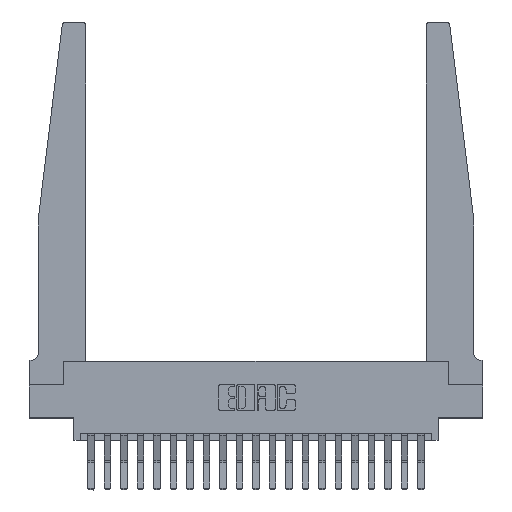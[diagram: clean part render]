
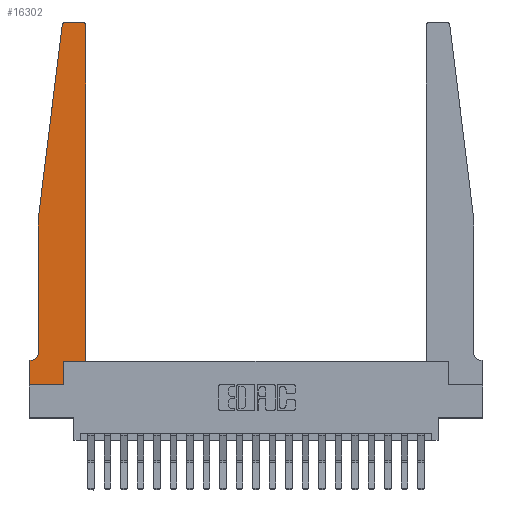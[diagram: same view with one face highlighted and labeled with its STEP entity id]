
A CAD part, top view. The second image highlights one B-rep face of the part: STEP entity #16302.
In plain terms, the highlighted planar face has unit normal (0, 0, 1).
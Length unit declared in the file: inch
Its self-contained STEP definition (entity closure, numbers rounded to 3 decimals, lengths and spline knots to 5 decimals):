
#2 = CARTESIAN_POINT ( 'NONE',  ( 0.395, 2.72, 0.37 ) ) ;
#70 = ORIENTED_EDGE ( 'NONE', *, *, #5399, .T. ) ;
#332 = CARTESIAN_POINT ( 'NONE',  ( 0.015, 0.2375, 0.37 ) ) ;
#385 = DIRECTION ( 'NONE',  ( 1., 0., 0. ) ) ;
#706 = VECTOR ( 'NONE', #16317, 39.37008 ) ;
#836 = CARTESIAN_POINT ( 'NONE',  ( 0.065, 0.2375, 0.37 ) ) ;
#853 = DIRECTION ( 'NONE',  ( 0., -1., 0. ) ) ;
#1120 = LINE ( 'NONE', #12809, #9482 ) ;
#1611 = VERTEX_POINT ( 'NONE', #3954 ) ;
#1660 = DIRECTION ( 'NONE',  ( 1., 0., 0. ) ) ;
#1911 = VERTEX_POINT ( 'NONE', #16457 ) ;
#1987 = DIRECTION ( 'NONE',  ( -1., 0., 0. ) ) ;
#2037 = AXIS2_PLACEMENT_3D ( 'NONE', #4890, #6555, #18270 ) ;
#2272 = ORIENTED_EDGE ( 'NONE', *, *, #21224, .T. ) ;
#2497 = ORIENTED_EDGE ( 'NONE', *, *, #7414, .T. ) ;
#2918 = CARTESIAN_POINT ( 'NONE',  ( 0.25, 2.75, 0.37 ) ) ;
#2957 = AXIS2_PLACEMENT_3D ( 'NONE', #2, #11694, #1660 ) ;
#3828 = CARTESIAN_POINT ( 'NONE',  ( 0., 0., 0.37 ) ) ;
#3954 = CARTESIAN_POINT ( 'NONE',  ( 0.425, 2.72, 0.37 ) ) ;
#4432 = DIRECTION ( 'NONE',  ( 0., -1., 0. ) ) ;
#4563 = VECTOR ( 'NONE', #21106, 39.37008 ) ;
#4702 = LINE ( 'NONE', #2918, #9673 ) ;
#4890 = CARTESIAN_POINT ( 'NONE',  ( 0., 0.1875, 0.37 ) ) ;
#5037 = CIRCLE ( 'NONE', #17905, 0.03 ) ;
#5399 = EDGE_CURVE ( 'NONE', #1911, #17386, #9581, .T. ) ;
#5474 = DIRECTION ( 'NONE',  ( 1., 0., 0. ) ) ;
#5552 = ORIENTED_EDGE ( 'NONE', *, *, #10979, .T. ) ;
#5596 = EDGE_CURVE ( 'NONE', #18341, #21487, #6407, .T. ) ;
#6071 = CARTESIAN_POINT ( 'NONE',  ( 0.015, 0.1875, 0.37 ) ) ;
#6191 = EDGE_LOOP ( 'NONE', ( #6474, #9960, #16438, #13829, #2497, #7590, #21113, #16544, #5552, #70, #2272, #18948 ) ) ;
#6401 = LINE ( 'NONE', #3828, #15356 ) ;
#6404 = DIRECTION ( 'NONE',  ( 0., 1., 0. ) ) ;
#6407 = LINE ( 'NONE', #18411, #10391 ) ;
#6474 = ORIENTED_EDGE ( 'NONE', *, *, #10945, .T. ) ;
#6555 = DIRECTION ( 'NONE',  ( 0., 0., 1. ) ) ;
#6981 = VERTEX_POINT ( 'NONE', #10583 ) ;
#7071 = CARTESIAN_POINT ( 'NONE',  ( 0.24675, 2.72367, 0.37 ) ) ;
#7397 = CARTESIAN_POINT ( 'NONE',  ( 0., 0.1875, 0.37 ) ) ;
#7414 = EDGE_CURVE ( 'NONE', #14392, #21229, #13473, .T. ) ;
#7590 = ORIENTED_EDGE ( 'NONE', *, *, #15091, .T. ) ;
#7788 = CARTESIAN_POINT ( 'NONE',  ( 0.065, 0.1875, 0.37 ) ) ;
#7789 = CIRCLE ( 'NONE', #2957, 0.03 ) ;
#7949 = DIRECTION ( 'NONE',  ( -1., 0., 0. ) ) ;
#8599 = LINE ( 'NONE', #14816, #20341 ) ;
#9482 = VECTOR ( 'NONE', #4432, 39.37008 ) ;
#9546 = DIRECTION ( 'NONE',  ( 0., 1., 0. ) ) ;
#9577 = CARTESIAN_POINT ( 'NONE',  ( 0.425, 0.18, 0.37 ) ) ;
#9581 = LINE ( 'NONE', #9577, #706 ) ;
#9673 = VECTOR ( 'NONE', #7949, 39.37008 ) ;
#9960 = ORIENTED_EDGE ( 'NONE', *, *, #20722, .T. ) ;
#10391 = VECTOR ( 'NONE', #20054, 39.37008 ) ;
#10399 = DIRECTION ( 'NONE',  ( 0., 0., 1. ) ) ;
#10583 = CARTESIAN_POINT ( 'NONE',  ( 0.2605, 0., 0.37 ) ) ;
#10895 = CARTESIAN_POINT ( 'NONE',  ( 0.065, 1.25, 0.37 ) ) ;
#10945 = EDGE_CURVE ( 'NONE', #18394, #11528, #4702, .T. ) ;
#10979 = EDGE_CURVE ( 'NONE', #6981, #1911, #8599, .T. ) ;
#11528 = VERTEX_POINT ( 'NONE', #17809 ) ;
#11694 = DIRECTION ( 'NONE',  ( 0., 0., 1. ) ) ;
#11712 = EDGE_CURVE ( 'NONE', #1611, #18394, #7789, .T. ) ;
#11841 = CARTESIAN_POINT ( 'NONE',  ( 0.065, 1.25, 0.37 ) ) ;
#12038 = DIRECTION ( 'NONE',  ( 0., 0., -1. ) ) ;
#12809 = CARTESIAN_POINT ( 'NONE',  ( 0., 0., 0.37 ) ) ;
#13449 = LINE ( 'NONE', #21161, #13964 ) ;
#13473 = CIRCLE ( 'NONE', #16330, 0.05 ) ;
#13829 = ORIENTED_EDGE ( 'NONE', *, *, #17236, .T. ) ;
#13964 = VECTOR ( 'NONE', #9546, 39.37008 ) ;
#14100 = VECTOR ( 'NONE', #853, 39.37008 ) ;
#14214 = EDGE_CURVE ( 'NONE', #17655, #6981, #6401, .T. ) ;
#14392 = VERTEX_POINT ( 'NONE', #836 ) ;
#14816 = CARTESIAN_POINT ( 'NONE',  ( 0.2605, 0.18, 0.37 ) ) ;
#14953 = PLANE ( 'NONE',  #2037 ) ;
#15091 = EDGE_CURVE ( 'NONE', #21229, #19077, #18922, .T. ) ;
#15356 = VECTOR ( 'NONE', #5474, 39.37008 ) ;
#16302 = ADVANCED_FACE ( 'NONE', ( #17069 ), #14953, .T. ) ;
#16317 = DIRECTION ( 'NONE',  ( 1., 0., 0. ) ) ;
#16330 = AXIS2_PLACEMENT_3D ( 'NONE', #332, #12038, #1987 ) ;
#16438 = ORIENTED_EDGE ( 'NONE', *, *, #5596, .T. ) ;
#16457 = CARTESIAN_POINT ( 'NONE',  ( 0.2605, 0.18, 0.37 ) ) ;
#16544 = ORIENTED_EDGE ( 'NONE', *, *, #14214, .T. ) ;
#17069 = FACE_OUTER_BOUND ( 'NONE', #6191, .T. ) ;
#17236 = EDGE_CURVE ( 'NONE', #21487, #14392, #18499, .T. ) ;
#17386 = VERTEX_POINT ( 'NONE', #21146 ) ;
#17655 = VERTEX_POINT ( 'NONE', #20218 ) ;
#17809 = CARTESIAN_POINT ( 'NONE',  ( 0.27653, 2.75, 0.37 ) ) ;
#17905 = AXIS2_PLACEMENT_3D ( 'NONE', #20328, #10399, #385 ) ;
#18270 = DIRECTION ( 'NONE',  ( 1., 0., 0. ) ) ;
#18341 = VERTEX_POINT ( 'NONE', #7071 ) ;
#18394 = VERTEX_POINT ( 'NONE', #18974 ) ;
#18411 = CARTESIAN_POINT ( 'NONE',  ( 0.065, 1.25, 0.37 ) ) ;
#18499 = LINE ( 'NONE', #10895, #14100 ) ;
#18922 = LINE ( 'NONE', #7788, #4563 ) ;
#18948 = ORIENTED_EDGE ( 'NONE', *, *, #11712, .T. ) ;
#18974 = CARTESIAN_POINT ( 'NONE',  ( 0.395, 2.75, 0.37 ) ) ;
#19077 = VERTEX_POINT ( 'NONE', #7397 ) ;
#20054 = DIRECTION ( 'NONE',  ( -0.122, -0.992, 0. ) ) ;
#20218 = CARTESIAN_POINT ( 'NONE',  ( 0., 0., 0.37 ) ) ;
#20328 = CARTESIAN_POINT ( 'NONE',  ( 0.27653, 2.72, 0.37 ) ) ;
#20341 = VECTOR ( 'NONE', #6404, 39.37008 ) ;
#20722 = EDGE_CURVE ( 'NONE', #11528, #18341, #5037, .T. ) ;
#21106 = DIRECTION ( 'NONE',  ( -1., 0., 0. ) ) ;
#21113 = ORIENTED_EDGE ( 'NONE', *, *, #21197, .T. ) ;
#21146 = CARTESIAN_POINT ( 'NONE',  ( 0.425, 0.18, 0.37 ) ) ;
#21161 = CARTESIAN_POINT ( 'NONE',  ( 0.425, 0.18, 0.37 ) ) ;
#21197 = EDGE_CURVE ( 'NONE', #19077, #17655, #1120, .T. ) ;
#21224 = EDGE_CURVE ( 'NONE', #17386, #1611, #13449, .T. ) ;
#21229 = VERTEX_POINT ( 'NONE', #6071 ) ;
#21487 = VERTEX_POINT ( 'NONE', #11841 ) ;
